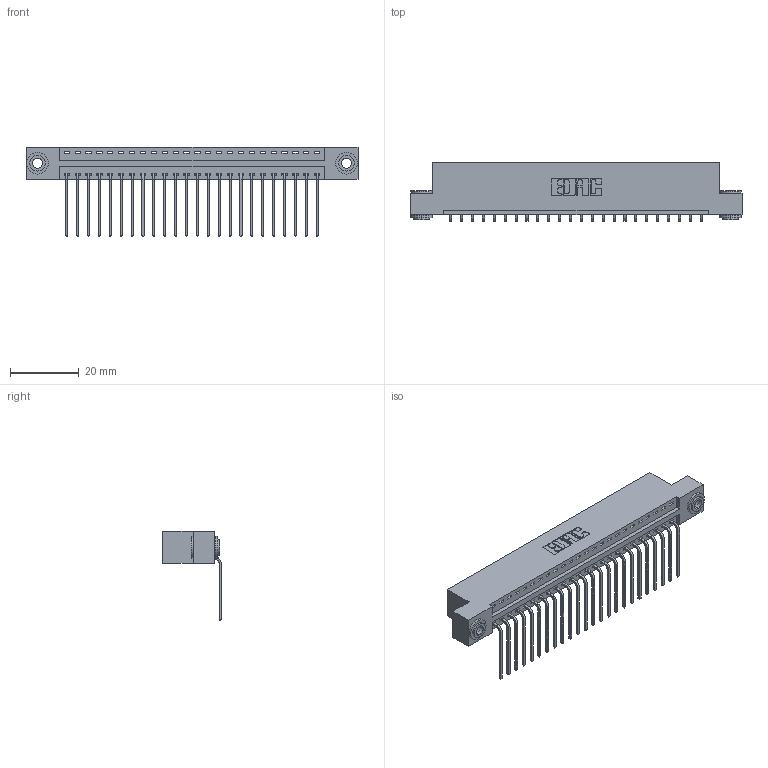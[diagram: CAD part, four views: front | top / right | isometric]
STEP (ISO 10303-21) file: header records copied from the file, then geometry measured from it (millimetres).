
FILE_DESCRIPTION (( 'STEP AP203' ), '1' );
FILE_NAME ('396-024-559-103.STEP', '2018-09-01T15:19:11', ( '' ), ( '' ), 'SwSTEP 2.0', 'SolidWorks 2016', '' );
FILE_SCHEMA (( 'CONFIG_CONTROL_DESIGN' ));
Length unit declared in the file: inch
Products named in the file (4): 346 Part_Flush Mounting Lugs - 0.156 Dia-TH; 345-292-001_558 559 Tail - 1; 345-250-002_345-250-002-102; 396-024-559-103
Assembly tree (27 placements, depth 2):
  396-024-559-103
    346 Part_Flush Mounting Lugs - 0.156 Dia-TH
    345-292-001_558 559 Tail - 1  x24
    345-250-002_345-250-002-102  x2
Bounding box: 96.77 x 17.08 x 26.16 mm (x, y, z)
Volume: 9238.8 mm3; surface area: 12049.2 mm2
Topology: 27 solids, 27 shells, 1600 faces, 4773 edges, 3146 vertices
Faces by surface type: plane 1094, cylinder 498, cone 8
Entity records: 18052 total; most frequent: CARTESIAN_POINT 3079, ORIENTED_EDGE 3030, DIRECTION 2769, EDGE_CURVE 1515, VECTOR 1263, LINE 1263, VERTEX_POINT 1006, AXIS2_PLACEMENT_3D 753
